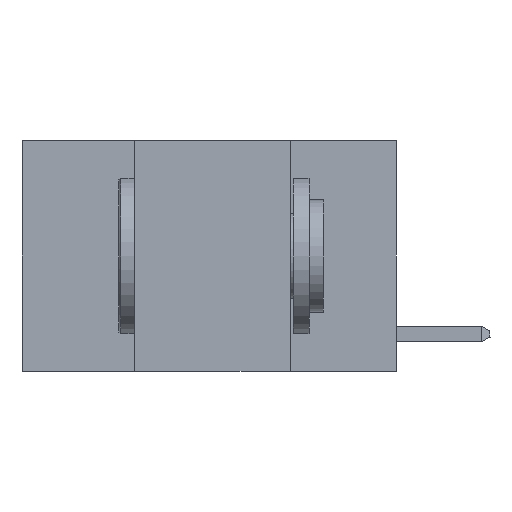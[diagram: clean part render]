
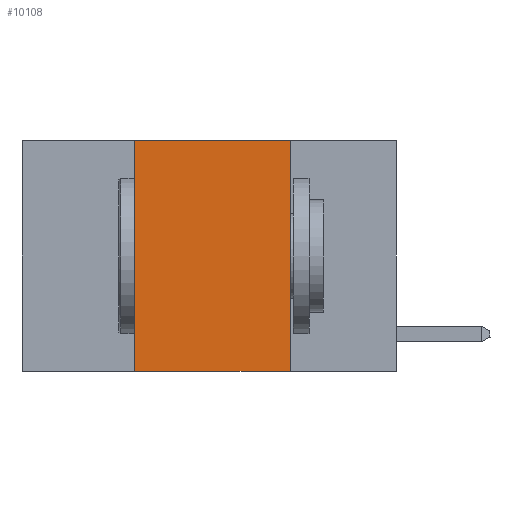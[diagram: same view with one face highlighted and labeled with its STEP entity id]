
A CAD part, left-side view. The second image highlights one B-rep face of the part: STEP entity #10108.
In plain terms, the highlighted planar face has unit normal (-1, 0, 0).
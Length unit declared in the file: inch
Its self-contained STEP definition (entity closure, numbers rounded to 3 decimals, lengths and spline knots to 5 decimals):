
#1640 = VERTEX_POINT ( 'NONE', #2954 ) ;
#1809 = LINE ( 'NONE', #7987, #5538 ) ;
#2194 = EDGE_CURVE ( 'NONE', #12813, #1640, #6689, .T. ) ;
#2954 = CARTESIAN_POINT ( 'NONE',  ( 0., 0.17, -0.37 ) ) ;
#3281 = DIRECTION ( 'NONE',  ( 0., -1., 0. ) ) ;
#3483 = VERTEX_POINT ( 'NONE', #13170 ) ;
#4138 = VECTOR ( 'NONE', #12933, 39.37008 ) ;
#4500 = AXIS2_PLACEMENT_3D ( 'NONE', #15932, #13658, #5709 ) ;
#4720 = VECTOR ( 'NONE', #3281, 39.37008 ) ;
#4976 = CARTESIAN_POINT ( 'NONE',  ( 0., 0.42, -0.37 ) ) ;
#5298 = DIRECTION ( 'NONE',  ( 0., 0., -1. ) ) ;
#5538 = VECTOR ( 'NONE', #17318, 39.37008 ) ;
#5709 = DIRECTION ( 'NONE',  ( 0., 0., -1. ) ) ;
#6313 = CARTESIAN_POINT ( 'NONE',  ( 0., 0.17, 0. ) ) ;
#6464 = ORIENTED_EDGE ( 'NONE', *, *, #12846, .F. ) ;
#6658 = EDGE_LOOP ( 'NONE', ( #8752, #9169, #6464, #9984 ) ) ;
#6689 = LINE ( 'NONE', #13272, #9786 ) ;
#7987 = CARTESIAN_POINT ( 'NONE',  ( 0., 0.6, -0.37 ) ) ;
#8536 = EDGE_CURVE ( 'NONE', #3483, #12813, #15416, .T. ) ;
#8752 = ORIENTED_EDGE ( 'NONE', *, *, #2194, .F. ) ;
#9169 = ORIENTED_EDGE ( 'NONE', *, *, #8536, .F. ) ;
#9786 = VECTOR ( 'NONE', #5298, 39.37008 ) ;
#9984 = ORIENTED_EDGE ( 'NONE', *, *, #14078, .T. ) ;
#10108 = ADVANCED_FACE ( 'NONE', ( #15795 ), #11961, .F. ) ;
#11335 = LINE ( 'NONE', #17038, #4138 ) ;
#11961 = PLANE ( 'NONE',  #4500 ) ;
#12813 = VERTEX_POINT ( 'NONE', #6313 ) ;
#12846 = EDGE_CURVE ( 'NONE', #17355, #3483, #11335, .T. ) ;
#12933 = DIRECTION ( 'NONE',  ( 0., 0., 1. ) ) ;
#13170 = CARTESIAN_POINT ( 'NONE',  ( 0., 0.42, 0. ) ) ;
#13272 = CARTESIAN_POINT ( 'NONE',  ( 0., 0.17, 0. ) ) ;
#13658 = DIRECTION ( 'NONE',  ( 1., 0., 0. ) ) ;
#13966 = CARTESIAN_POINT ( 'NONE',  ( 0., 0.6, 0. ) ) ;
#14078 = EDGE_CURVE ( 'NONE', #17355, #1640, #1809, .T. ) ;
#15416 = LINE ( 'NONE', #13966, #4720 ) ;
#15795 = FACE_OUTER_BOUND ( 'NONE', #6658, .T. ) ;
#15932 = CARTESIAN_POINT ( 'NONE',  ( 0., 0.6, 0. ) ) ;
#17038 = CARTESIAN_POINT ( 'NONE',  ( 0., 0.42, 0. ) ) ;
#17318 = DIRECTION ( 'NONE',  ( 0., -1., 0. ) ) ;
#17355 = VERTEX_POINT ( 'NONE', #4976 ) ;
